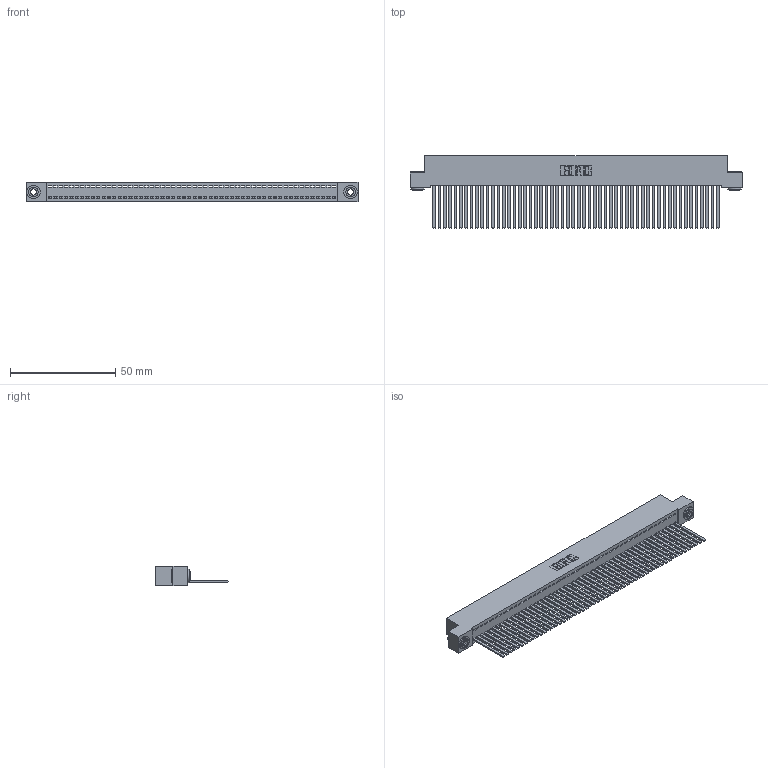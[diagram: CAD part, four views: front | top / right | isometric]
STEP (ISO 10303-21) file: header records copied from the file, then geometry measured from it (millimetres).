
FILE_DESCRIPTION (( 'STEP AP203' ), '1' );
FILE_NAME ('342-054-544-103.STEP', '2019-10-03T03:22:46', ( '' ), ( '' ), 'SwSTEP 2.0', 'SolidWorks 2016', '' );
FILE_SCHEMA (( 'CONFIG_CONTROL_DESIGN' ));
Length unit declared in the file: inch
Products named in the file (4): 342 Part_.156 TH; 345-292-001_345-293-144; 342-250-002_345-250-002-102; 342-054-544-103
Assembly tree (57 placements, depth 2):
  342-054-544-103
    342 Part_.156 TH
    345-292-001_345-293-144  x54
    342-250-002_345-250-002-102  x2
Bounding box: 157.48 x 34.3 x 9.4 mm (x, y, z)
Volume: 14500.3 mm3; surface area: 23523.1 mm2
Topology: 57 solids, 57 shells, 2956 faces, 8907 edges, 5862 vertices
Faces by surface type: plane 2128, cylinder 820, cone 8
Entity records: 31794 total; most frequent: CARTESIAN_POINT 5459, ORIENTED_EDGE 5442, DIRECTION 4611, EDGE_CURVE 2721, VECTOR 2573, LINE 2573, VERTEX_POINT 1810, AXIS2_PLACEMENT_3D 1019
